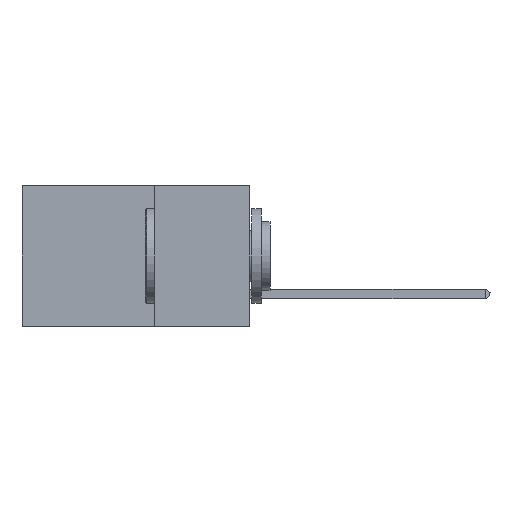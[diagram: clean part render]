
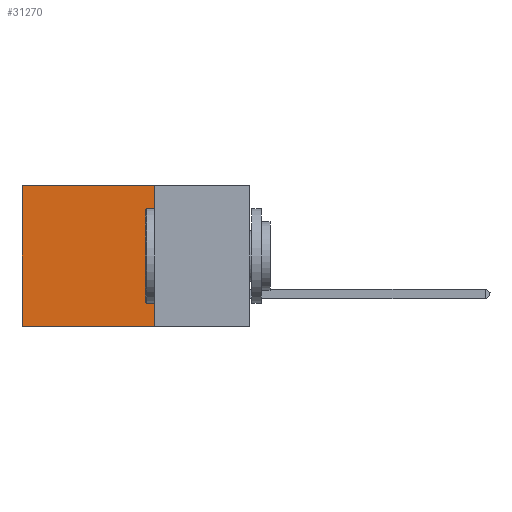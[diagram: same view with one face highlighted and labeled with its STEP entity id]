
A CAD part, left-side view. The second image highlights one B-rep face of the part: STEP entity #31270.
In plain terms, the highlighted planar face has unit normal (-1, 0, 0).
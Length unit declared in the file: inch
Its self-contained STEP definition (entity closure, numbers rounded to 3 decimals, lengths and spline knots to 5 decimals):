
#328 = VECTOR ( 'NONE', #5488, 39.37008 ) ;
#541 = FACE_OUTER_BOUND ( 'NONE', #21774, .T. ) ;
#635 = EDGE_CURVE ( 'NONE', #12425, #38788, #28096, .T. ) ;
#1962 = CARTESIAN_POINT ( 'NONE',  ( 0.2875, 0.25, 0. ) ) ;
#2148 = PLANE ( 'NONE',  #30392 ) ;
#5488 = DIRECTION ( 'NONE',  ( 0., 1., 0. ) ) ;
#6168 = DIRECTION ( 'NONE',  ( 1., 0., 0. ) ) ;
#10668 = EDGE_CURVE ( 'NONE', #12425, #33440, #14311, .T. ) ;
#12173 = CARTESIAN_POINT ( 'NONE',  ( 0.2875, 0.25, 0. ) ) ;
#12425 = VERTEX_POINT ( 'NONE', #29315 ) ;
#14311 = LINE ( 'NONE', #48032, #23617 ) ;
#16845 = CARTESIAN_POINT ( 'NONE',  ( 0.2875, 0.6, -0.37 ) ) ;
#17882 = ORIENTED_EDGE ( 'NONE', *, *, #10668, .F. ) ;
#20422 = DIRECTION ( 'NONE',  ( 0., 0., -1. ) ) ;
#21774 = EDGE_LOOP ( 'NONE', ( #45879, #41330, #17882, #26757 ) ) ;
#22610 = EDGE_CURVE ( 'NONE', #33440, #40463, #47144, .T. ) ;
#22989 = VECTOR ( 'NONE', #20422, 39.37008 ) ;
#23617 = VECTOR ( 'NONE', #48207, 39.37008 ) ;
#24734 = CARTESIAN_POINT ( 'NONE',  ( 0.2875, 0.25, -0.37 ) ) ;
#26757 = ORIENTED_EDGE ( 'NONE', *, *, #635, .T. ) ;
#28096 = LINE ( 'NONE', #12173, #328 ) ;
#28567 = DIRECTION ( 'NONE',  ( 0., 0., -1. ) ) ;
#29315 = CARTESIAN_POINT ( 'NONE',  ( 0.2875, 0.25, 0. ) ) ;
#29479 = VECTOR ( 'NONE', #34224, 39.37008 ) ;
#29767 = CARTESIAN_POINT ( 'NONE',  ( 0.2875, 0.6, 0. ) ) ;
#30392 = AXIS2_PLACEMENT_3D ( 'NONE', #1962, #6168, #28567 ) ;
#31270 = ADVANCED_FACE ( 'NONE', ( #541 ), #2148, .F. ) ;
#32793 = EDGE_CURVE ( 'NONE', #38788, #40463, #43037, .T. ) ;
#33440 = VERTEX_POINT ( 'NONE', #24734 ) ;
#34224 = DIRECTION ( 'NONE',  ( 0., 1., 0. ) ) ;
#38788 = VERTEX_POINT ( 'NONE', #40562 ) ;
#40463 = VERTEX_POINT ( 'NONE', #16845 ) ;
#40562 = CARTESIAN_POINT ( 'NONE',  ( 0.2875, 0.6, 0. ) ) ;
#41330 = ORIENTED_EDGE ( 'NONE', *, *, #22610, .F. ) ;
#42804 = CARTESIAN_POINT ( 'NONE',  ( 0.2875, 0.25, -0.37 ) ) ;
#43037 = LINE ( 'NONE', #29767, #22989 ) ;
#45879 = ORIENTED_EDGE ( 'NONE', *, *, #32793, .T. ) ;
#47144 = LINE ( 'NONE', #42804, #29479 ) ;
#48032 = CARTESIAN_POINT ( 'NONE',  ( 0.2875, 0.25, 0. ) ) ;
#48207 = DIRECTION ( 'NONE',  ( 0., 0., -1. ) ) ;
